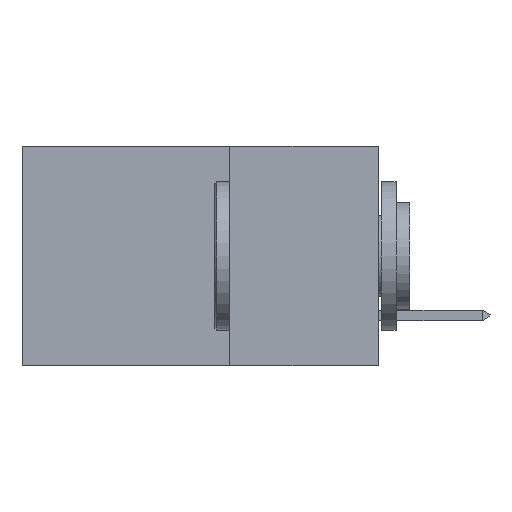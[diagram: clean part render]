
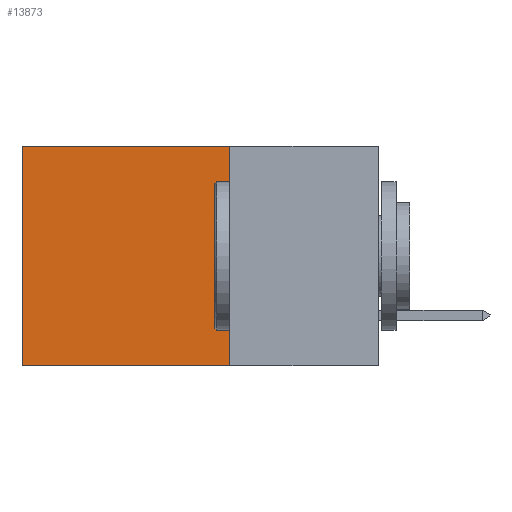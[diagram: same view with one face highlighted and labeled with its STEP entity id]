
A CAD part, left-side view. The second image highlights one B-rep face of the part: STEP entity #13873.
In plain terms, the highlighted planar face has unit normal (-1, 0, 0).
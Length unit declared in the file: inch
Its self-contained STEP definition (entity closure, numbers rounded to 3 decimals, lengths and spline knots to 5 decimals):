
#4309 = CARTESIAN_POINT ( 'NONE',  ( 0.298, 0.25, -0.37 ) ) ;
#4970 = VERTEX_POINT ( 'NONE', #4309 ) ;
#5421 = VECTOR ( 'NONE', #13068, 39.37008 ) ;
#6660 = AXIS2_PLACEMENT_3D ( 'NONE', #8997, #25923, #28577 ) ;
#7012 = EDGE_CURVE ( 'NONE', #4970, #10393, #8434, .T. ) ;
#8434 = LINE ( 'NONE', #30516, #23226 ) ;
#8997 = CARTESIAN_POINT ( 'NONE',  ( 0.298, 0.25, 0. ) ) ;
#9464 = VERTEX_POINT ( 'NONE', #25634 ) ;
#10393 = VERTEX_POINT ( 'NONE', #15754 ) ;
#11322 = LINE ( 'NONE', #20728, #17411 ) ;
#11509 = ORIENTED_EDGE ( 'NONE', *, *, #22192, .T. ) ;
#11888 = LINE ( 'NONE', #27547, #5421 ) ;
#13068 = DIRECTION ( 'NONE',  ( 0., 1., 0. ) ) ;
#13256 = ORIENTED_EDGE ( 'NONE', *, *, #7012, .F. ) ;
#13873 = ADVANCED_FACE ( 'NONE', ( #29294 ), #23499, .F. ) ;
#15754 = CARTESIAN_POINT ( 'NONE',  ( 0.298, 0.6, -0.37 ) ) ;
#17411 = VECTOR ( 'NONE', #20427, 39.37008 ) ;
#17503 = VECTOR ( 'NONE', #30767, 39.37008 ) ;
#17936 = ORIENTED_EDGE ( 'NONE', *, *, #23709, .F. ) ;
#18532 = CARTESIAN_POINT ( 'NONE',  ( 0.298, 0.6, 0. ) ) ;
#18940 = CARTESIAN_POINT ( 'NONE',  ( 0.298, 0.6, 0. ) ) ;
#20427 = DIRECTION ( 'NONE',  ( 0., 0., -1. ) ) ;
#20728 = CARTESIAN_POINT ( 'NONE',  ( 0.298, 0.25, 0. ) ) ;
#22192 = EDGE_CURVE ( 'NONE', #28697, #10393, #29592, .T. ) ;
#23226 = VECTOR ( 'NONE', #27988, 39.37008 ) ;
#23499 = PLANE ( 'NONE',  #6660 ) ;
#23709 = EDGE_CURVE ( 'NONE', #9464, #4970, #11322, .T. ) ;
#25634 = CARTESIAN_POINT ( 'NONE',  ( 0.298, 0.25, 0. ) ) ;
#25923 = DIRECTION ( 'NONE',  ( 1., 0., 0. ) ) ;
#26077 = ORIENTED_EDGE ( 'NONE', *, *, #26275, .T. ) ;
#26275 = EDGE_CURVE ( 'NONE', #9464, #28697, #11888, .T. ) ;
#27547 = CARTESIAN_POINT ( 'NONE',  ( 0.298, 0.25, 0. ) ) ;
#27988 = DIRECTION ( 'NONE',  ( 0., 1., 0. ) ) ;
#28577 = DIRECTION ( 'NONE',  ( 0., 0., -1. ) ) ;
#28697 = VERTEX_POINT ( 'NONE', #18940 ) ;
#29113 = EDGE_LOOP ( 'NONE', ( #11509, #13256, #17936, #26077 ) ) ;
#29294 = FACE_OUTER_BOUND ( 'NONE', #29113, .T. ) ;
#29592 = LINE ( 'NONE', #18532, #17503 ) ;
#30516 = CARTESIAN_POINT ( 'NONE',  ( 0.298, 0.25, -0.37 ) ) ;
#30767 = DIRECTION ( 'NONE',  ( 0., 0., -1. ) ) ;
